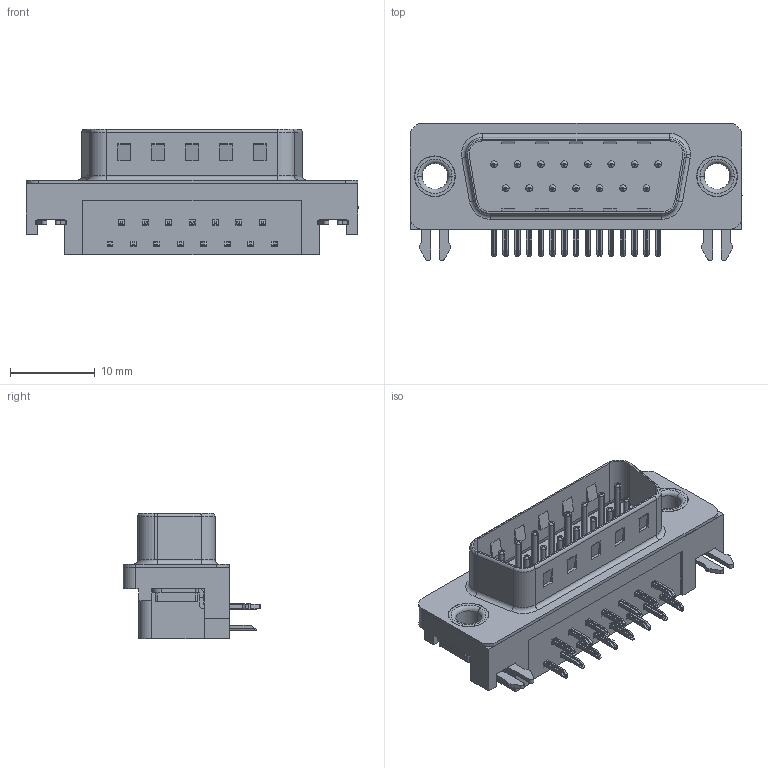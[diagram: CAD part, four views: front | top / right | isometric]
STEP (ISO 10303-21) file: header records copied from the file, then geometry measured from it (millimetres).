
FILE_DESCRIPTION (( 'STEP AP203' ), '1' );
FILE_NAME ('623-015-261-031.STEP', '2018-11-06T12:16:23', ( '' ), ( '' ), 'SwSTEP 2.0', 'SolidWorks 2016', '' );
FILE_SCHEMA (( 'CONFIG_CONTROL_DESIGN' ));
Length unit declared in the file: millimetre
Products named in the file (7): 623 Housing_15 Socket; 623 Shell_15 Socket; 623 Contact Bottom; 623 Contact Top; 623 2 Prong Board Lock; 623 Thru Hole Rivet; 623-015-261-031
Assembly tree (21 placements, depth 2):
  623-015-261-031
    623 Housing_15 Socket
    623 Shell_15 Socket
    623 Contact Bottom  x7
    623 Contact Top  x8
    623 2 Prong Board Lock  x2
    623 Thru Hole Rivet  x2
Bounding box: 39.22 x 16.25 x 14.8 mm (x, y, z)
Volume: 3314.7 mm3; surface area: 4923.2 mm2
Topology: 21 solids, 21 shells, 1459 faces, 3621 edges, 2245 vertices
Faces by surface type: plane 921, cylinder 421, torus 117
Entity records: 16785 total; most frequent: DIRECTION 2764, CARTESIAN_POINT 2721, ORIENTED_EDGE 2616, EDGE_CURVE 1308, VECTOR 928, LINE 928, AXIS2_PLACEMENT_3D 918, VERTEX_POINT 835
